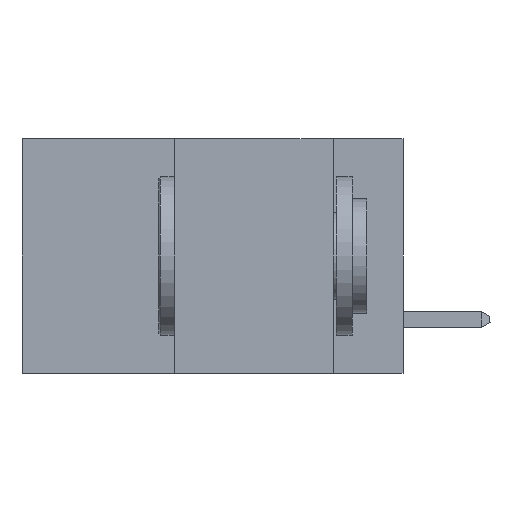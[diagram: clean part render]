
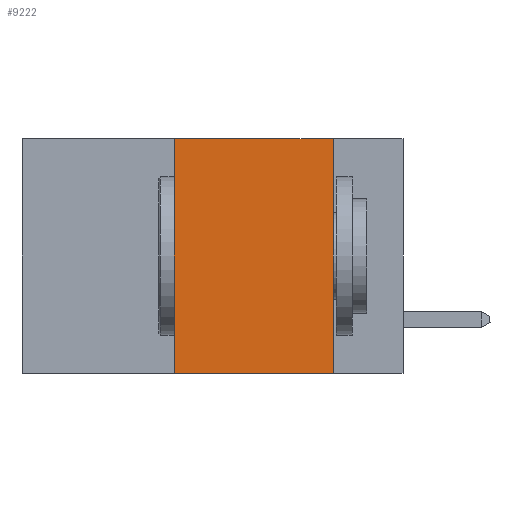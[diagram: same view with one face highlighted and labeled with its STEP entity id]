
A CAD part, left-side view. The second image highlights one B-rep face of the part: STEP entity #9222.
In plain terms, the highlighted planar face has unit normal (-1, 0, 0).
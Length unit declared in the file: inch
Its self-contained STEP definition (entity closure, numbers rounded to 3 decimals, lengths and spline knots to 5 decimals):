
#143 = LINE ( 'NONE', #16604, #13677 ) ;
#176 = VECTOR ( 'NONE', #1716, 39.37008 ) ;
#1121 = EDGE_CURVE ( 'NONE', #10748, #2482, #11653, .T. ) ;
#1143 = ORIENTED_EDGE ( 'NONE', *, *, #6554, .F. ) ;
#1561 = VERTEX_POINT ( 'NONE', #3686 ) ;
#1584 = EDGE_CURVE ( 'NONE', #2482, #1561, #143, .T. ) ;
#1716 = DIRECTION ( 'NONE',  ( 0., 0., 1. ) ) ;
#2268 = EDGE_CURVE ( 'NONE', #10748, #7228, #15506, .T. ) ;
#2482 = VERTEX_POINT ( 'NONE', #4982 ) ;
#3526 = PLANE ( 'NONE',  #3584 ) ;
#3584 = AXIS2_PLACEMENT_3D ( 'NONE', #14175, #3792, #11712 ) ;
#3686 = CARTESIAN_POINT ( 'NONE',  ( 0., 0.11, 0. ) ) ;
#3792 = DIRECTION ( 'NONE',  ( 1., 0., 0. ) ) ;
#4081 = FACE_OUTER_BOUND ( 'NONE', #5230, .T. ) ;
#4459 = CARTESIAN_POINT ( 'NONE',  ( 0., 0.11, -0.37 ) ) ;
#4982 = CARTESIAN_POINT ( 'NONE',  ( 0., 0.36, 0. ) ) ;
#5230 = EDGE_LOOP ( 'NONE', ( #1143, #9261, #10310, #7487 ) ) ;
#6380 = CARTESIAN_POINT ( 'NONE',  ( 0., 0.11, 0. ) ) ;
#6554 = EDGE_CURVE ( 'NONE', #1561, #7228, #14668, .T. ) ;
#6688 = DIRECTION ( 'NONE',  ( 0., -1., 0. ) ) ;
#7228 = VERTEX_POINT ( 'NONE', #4459 ) ;
#7487 = ORIENTED_EDGE ( 'NONE', *, *, #2268, .T. ) ;
#9222 = ADVANCED_FACE ( 'NONE', ( #4081 ), #3526, .F. ) ;
#9261 = ORIENTED_EDGE ( 'NONE', *, *, #1584, .F. ) ;
#10310 = ORIENTED_EDGE ( 'NONE', *, *, #1121, .F. ) ;
#10558 = CARTESIAN_POINT ( 'NONE',  ( 0., 0.36, -0.37 ) ) ;
#10748 = VERTEX_POINT ( 'NONE', #10558 ) ;
#11653 = LINE ( 'NONE', #16089, #176 ) ;
#11712 = DIRECTION ( 'NONE',  ( 0., 0., -1. ) ) ;
#13040 = VECTOR ( 'NONE', #14238, 39.37008 ) ;
#13677 = VECTOR ( 'NONE', #6688, 39.37008 ) ;
#14175 = CARTESIAN_POINT ( 'NONE',  ( 0., 0.6, 0. ) ) ;
#14238 = DIRECTION ( 'NONE',  ( 0., 0., -1. ) ) ;
#14668 = LINE ( 'NONE', #6380, #13040 ) ;
#14965 = CARTESIAN_POINT ( 'NONE',  ( 0., 0.6, -0.37 ) ) ;
#15024 = DIRECTION ( 'NONE',  ( 0., -1., 0. ) ) ;
#15506 = LINE ( 'NONE', #14965, #15711 ) ;
#15711 = VECTOR ( 'NONE', #15024, 39.37008 ) ;
#16089 = CARTESIAN_POINT ( 'NONE',  ( 0., 0.36, 0. ) ) ;
#16604 = CARTESIAN_POINT ( 'NONE',  ( 0., 0.6, 0. ) ) ;
